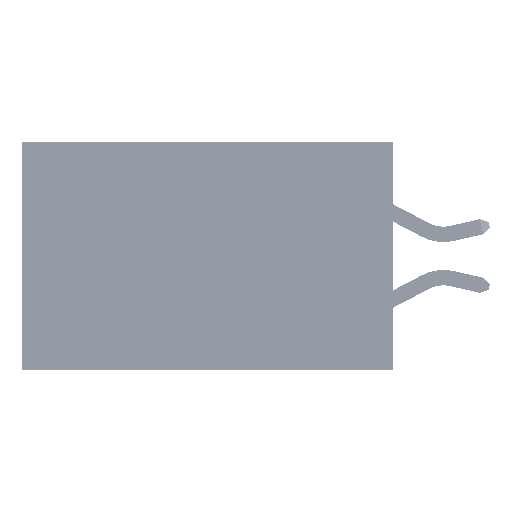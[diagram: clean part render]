
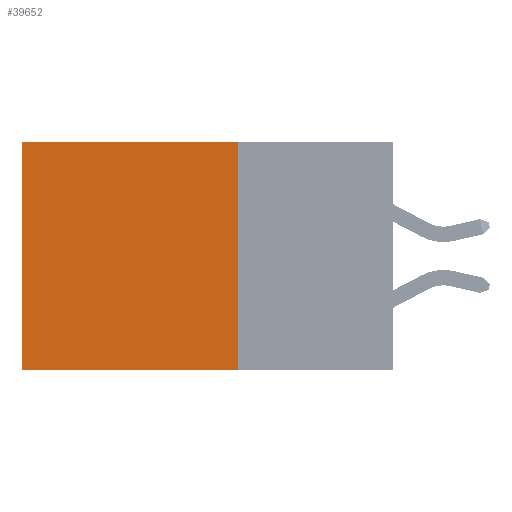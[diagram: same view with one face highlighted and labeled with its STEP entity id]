
A CAD part, left-side view. The second image highlights one B-rep face of the part: STEP entity #39652.
In plain terms, the highlighted planar face has unit normal (-1, 0, 0).
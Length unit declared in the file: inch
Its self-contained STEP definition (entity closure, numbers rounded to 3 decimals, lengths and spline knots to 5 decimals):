
#2761 = EDGE_CURVE ( 'NONE', #29992, #16555, #24301, .T. ) ;
#3160 = CARTESIAN_POINT ( 'NONE',  ( 0.2875, 0.6, 0. ) ) ;
#4115 = CARTESIAN_POINT ( 'NONE',  ( 0.2875, 0.25, -0.37 ) ) ;
#4659 = CARTESIAN_POINT ( 'NONE',  ( 0.2875, 0.6, -0.37 ) ) ;
#5404 = CARTESIAN_POINT ( 'NONE',  ( 0.2875, 0.25, -0.37 ) ) ;
#5670 = DIRECTION ( 'NONE',  ( 0., 0., -1. ) ) ;
#6177 = EDGE_CURVE ( 'NONE', #16555, #31737, #17130, .T. ) ;
#8858 = PLANE ( 'NONE',  #24501 ) ;
#11145 = VECTOR ( 'NONE', #5670, 39.37008 ) ;
#12188 = DIRECTION ( 'NONE',  ( 0., 1., 0. ) ) ;
#13240 = VECTOR ( 'NONE', #20222, 39.37008 ) ;
#15783 = CARTESIAN_POINT ( 'NONE',  ( 0.2875, 0.25, 0. ) ) ;
#15974 = CARTESIAN_POINT ( 'NONE',  ( 0.2875, 0.25, 0. ) ) ;
#16410 = EDGE_CURVE ( 'NONE', #29992, #25575, #35973, .T. ) ;
#16555 = VERTEX_POINT ( 'NONE', #4115 ) ;
#16682 = DIRECTION ( 'NONE',  ( 0., 1., 0. ) ) ;
#17130 = LINE ( 'NONE', #5404, #23954 ) ;
#18905 = DIRECTION ( 'NONE',  ( 0., 0., -1. ) ) ;
#19718 = ORIENTED_EDGE ( 'NONE', *, *, #6177, .F. ) ;
#20222 = DIRECTION ( 'NONE',  ( 0., 0., -1. ) ) ;
#20307 = FACE_OUTER_BOUND ( 'NONE', #35179, .T. ) ;
#23954 = VECTOR ( 'NONE', #12188, 39.37008 ) ;
#24301 = LINE ( 'NONE', #28425, #13240 ) ;
#24501 = AXIS2_PLACEMENT_3D ( 'NONE', #15974, #36144, #18905 ) ;
#25261 = EDGE_CURVE ( 'NONE', #25575, #31737, #42254, .T. ) ;
#25575 = VERTEX_POINT ( 'NONE', #3160 ) ;
#27503 = VECTOR ( 'NONE', #16682, 39.37008 ) ;
#28425 = CARTESIAN_POINT ( 'NONE',  ( 0.2875, 0.25, 0. ) ) ;
#29992 = VERTEX_POINT ( 'NONE', #15783 ) ;
#30030 = ORIENTED_EDGE ( 'NONE', *, *, #16410, .T. ) ;
#31737 = VERTEX_POINT ( 'NONE', #4659 ) ;
#35179 = EDGE_LOOP ( 'NONE', ( #38906, #19718, #40163, #30030 ) ) ;
#35897 = CARTESIAN_POINT ( 'NONE',  ( 0.2875, 0.6, 0. ) ) ;
#35973 = LINE ( 'NONE', #43473, #27503 ) ;
#36144 = DIRECTION ( 'NONE',  ( 1., 0., 0. ) ) ;
#38906 = ORIENTED_EDGE ( 'NONE', *, *, #25261, .T. ) ;
#39652 = ADVANCED_FACE ( 'NONE', ( #20307 ), #8858, .F. ) ;
#40163 = ORIENTED_EDGE ( 'NONE', *, *, #2761, .F. ) ;
#42254 = LINE ( 'NONE', #35897, #11145 ) ;
#43473 = CARTESIAN_POINT ( 'NONE',  ( 0.2875, 0.25, 0. ) ) ;
